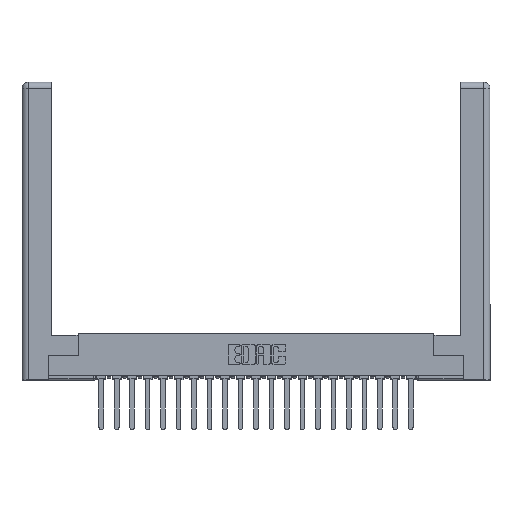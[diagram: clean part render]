
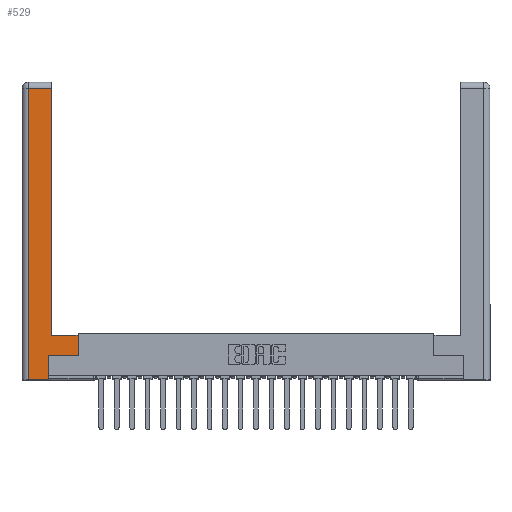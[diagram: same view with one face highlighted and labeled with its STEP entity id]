
A CAD part, top view. The second image highlights one B-rep face of the part: STEP entity #529.
In plain terms, the highlighted planar face has unit normal (0, 0, 1).
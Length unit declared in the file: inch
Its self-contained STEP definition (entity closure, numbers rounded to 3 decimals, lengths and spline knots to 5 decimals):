
#529 = ADVANCED_FACE ( 'NONE', ( #9066 ), #13049, .F. ) ;
#912 = LINE ( 'NONE', #8177, #12884 ) ;
#1380 = VERTEX_POINT ( 'NONE', #4167 ) ;
#2120 = CARTESIAN_POINT ( 'NONE',  ( 0.0615, 0., 0. ) ) ;
#2586 = VECTOR ( 'NONE', #7661, 39.37008 ) ;
#2680 = LINE ( 'NONE', #21676, #5699 ) ;
#2934 = VERTEX_POINT ( 'NONE', #16618 ) ;
#3079 = CARTESIAN_POINT ( 'NONE',  ( 0.565, 0.45, 0. ) ) ;
#3960 = LINE ( 'NONE', #2120, #22368 ) ;
#4167 = CARTESIAN_POINT ( 'NONE',  ( 0.0615, 0., 0. ) ) ;
#4406 = LINE ( 'NONE', #3079, #21203 ) ;
#4482 = VECTOR ( 'NONE', #18270, 39.37008 ) ;
#4776 = VERTEX_POINT ( 'NONE', #5937 ) ;
#5373 = CARTESIAN_POINT ( 'NONE',  ( 0.295, 3., 0. ) ) ;
#5699 = VECTOR ( 'NONE', #10061, 39.37008 ) ;
#5735 = LINE ( 'NONE', #5373, #2586 ) ;
#5880 = DIRECTION ( 'NONE',  ( 0., -1., 0. ) ) ;
#5937 = CARTESIAN_POINT ( 'NONE',  ( 0.565, 0.245, 0. ) ) ;
#5999 = DIRECTION ( 'NONE',  ( -1., 0., 0. ) ) ;
#6082 = DIRECTION ( 'NONE',  ( 1., 0., 0. ) ) ;
#6415 = EDGE_CURVE ( 'NONE', #22541, #10482, #9185, .T. ) ;
#7661 = DIRECTION ( 'NONE',  ( 0., 1., 0. ) ) ;
#7756 = CARTESIAN_POINT ( 'NONE',  ( 0.265, 0., 0. ) ) ;
#7935 = CARTESIAN_POINT ( 'NONE',  ( 0.295, 0.45, 0. ) ) ;
#8177 = CARTESIAN_POINT ( 'NONE',  ( 0.265, 0.245, 0. ) ) ;
#8178 = EDGE_CURVE ( 'NONE', #2934, #22541, #5735, .T. ) ;
#9053 = ORIENTED_EDGE ( 'NONE', *, *, #9189, .T. ) ;
#9066 = FACE_OUTER_BOUND ( 'NONE', #9196, .T. ) ;
#9185 = LINE ( 'NONE', #16314, #4482 ) ;
#9189 = EDGE_CURVE ( 'NONE', #10482, #1380, #3960, .T. ) ;
#9196 = EDGE_LOOP ( 'NONE', ( #23142, #23384, #9053, #17354, #10566, #11984, #19962, #12701 ) ) ;
#9392 = LINE ( 'NONE', #7935, #20247 ) ;
#10061 = DIRECTION ( 'NONE',  ( 1., 0., 0. ) ) ;
#10460 = VERTEX_POINT ( 'NONE', #22049 ) ;
#10482 = VERTEX_POINT ( 'NONE', #22402 ) ;
#10566 = ORIENTED_EDGE ( 'NONE', *, *, #17834, .T. ) ;
#11984 = ORIENTED_EDGE ( 'NONE', *, *, #16321, .T. ) ;
#12698 = CARTESIAN_POINT ( 'NONE',  ( 0., 0., 0. ) ) ;
#12701 = ORIENTED_EDGE ( 'NONE', *, *, #17688, .T. ) ;
#12884 = VECTOR ( 'NONE', #15538, 39.37008 ) ;
#13049 = PLANE ( 'NONE',  #18925 ) ;
#14444 = CARTESIAN_POINT ( 'NONE',  ( 0.295, 2.94, 0. ) ) ;
#14743 = DIRECTION ( 'NONE',  ( 0., 0., -1. ) ) ;
#15074 = CARTESIAN_POINT ( 'NONE',  ( 0.565, 0.45, 0. ) ) ;
#15538 = DIRECTION ( 'NONE',  ( 0., 1., 0. ) ) ;
#15769 = DIRECTION ( 'NONE',  ( 0., 1., 0. ) ) ;
#16314 = CARTESIAN_POINT ( 'NONE',  ( 0.0615, 2.94, 0. ) ) ;
#16321 = EDGE_CURVE ( 'NONE', #10460, #4776, #20864, .T. ) ;
#16448 = DIRECTION ( 'NONE',  ( -1., 0., 0. ) ) ;
#16618 = CARTESIAN_POINT ( 'NONE',  ( 0.295, 0.45, 0. ) ) ;
#16772 = VERTEX_POINT ( 'NONE', #7756 ) ;
#17092 = CARTESIAN_POINT ( 'NONE',  ( 0.565, 0.245, 0. ) ) ;
#17354 = ORIENTED_EDGE ( 'NONE', *, *, #22083, .T. ) ;
#17688 = EDGE_CURVE ( 'NONE', #19806, #2934, #9392, .T. ) ;
#17834 = EDGE_CURVE ( 'NONE', #16772, #10460, #912, .T. ) ;
#18270 = DIRECTION ( 'NONE',  ( -1., 0., 0. ) ) ;
#18925 = AXIS2_PLACEMENT_3D ( 'NONE', #12698, #14743, #16448 ) ;
#19806 = VERTEX_POINT ( 'NONE', #15074 ) ;
#19962 = ORIENTED_EDGE ( 'NONE', *, *, #22774, .T. ) ;
#20247 = VECTOR ( 'NONE', #5999, 39.37008 ) ;
#20864 = LINE ( 'NONE', #17092, #22930 ) ;
#21203 = VECTOR ( 'NONE', #15769, 39.37008 ) ;
#21676 = CARTESIAN_POINT ( 'NONE',  ( 0.265, 0., 0. ) ) ;
#22049 = CARTESIAN_POINT ( 'NONE',  ( 0.265, 0.245, 0. ) ) ;
#22083 = EDGE_CURVE ( 'NONE', #1380, #16772, #2680, .T. ) ;
#22368 = VECTOR ( 'NONE', #5880, 39.37008 ) ;
#22402 = CARTESIAN_POINT ( 'NONE',  ( 0.0615, 2.94, 0. ) ) ;
#22541 = VERTEX_POINT ( 'NONE', #14444 ) ;
#22774 = EDGE_CURVE ( 'NONE', #4776, #19806, #4406, .T. ) ;
#22930 = VECTOR ( 'NONE', #6082, 39.37008 ) ;
#23142 = ORIENTED_EDGE ( 'NONE', *, *, #8178, .T. ) ;
#23384 = ORIENTED_EDGE ( 'NONE', *, *, #6415, .T. ) ;
